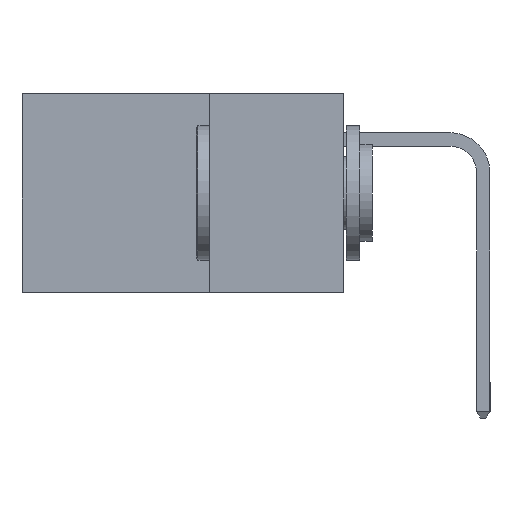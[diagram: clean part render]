
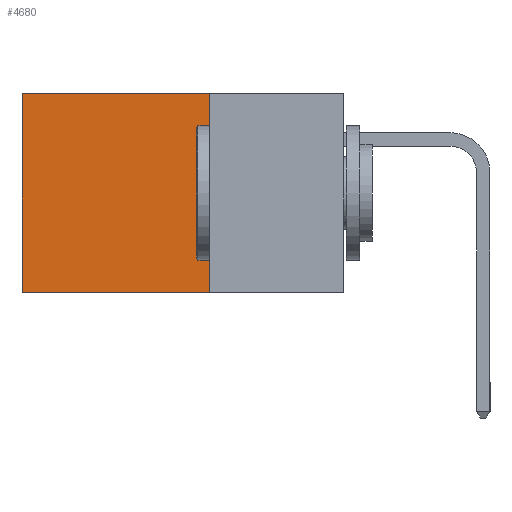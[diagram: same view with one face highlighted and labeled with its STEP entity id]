
A CAD part, left-side view. The second image highlights one B-rep face of the part: STEP entity #4680.
In plain terms, the highlighted planar face has unit normal (-1, 0, 0).
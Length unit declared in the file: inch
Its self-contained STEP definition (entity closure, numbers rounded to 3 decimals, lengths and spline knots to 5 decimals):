
#253 = CARTESIAN_POINT ( 'NONE',  ( 0.298, 0.6, 0. ) ) ;
#821 = VERTEX_POINT ( 'NONE', #8189 ) ;
#877 = ORIENTED_EDGE ( 'NONE', *, *, #25075, .F. ) ;
#981 = VERTEX_POINT ( 'NONE', #253 ) ;
#1596 = EDGE_CURVE ( 'NONE', #12907, #18561, #21260, .T. ) ;
#1654 = ORIENTED_EDGE ( 'NONE', *, *, #10712, .T. ) ;
#2031 = DIRECTION ( 'NONE',  ( 0., 1., 0. ) ) ;
#2987 = PLANE ( 'NONE',  #20745 ) ;
#3049 = CARTESIAN_POINT ( 'NONE',  ( 0.298, 0.6, 0. ) ) ;
#3614 = EDGE_CURVE ( 'NONE', #821, #981, #21253, .T. ) ;
#4680 = ADVANCED_FACE ( 'NONE', ( #14351 ), #2987, .F. ) ;
#4738 = CARTESIAN_POINT ( 'NONE',  ( 0.298, 0.25, -0.37 ) ) ;
#8189 = CARTESIAN_POINT ( 'NONE',  ( 0.298, 0.25, 0. ) ) ;
#8745 = LINE ( 'NONE', #3049, #18729 ) ;
#9806 = VECTOR ( 'NONE', #24701, 39.37008 ) ;
#10047 = VECTOR ( 'NONE', #12560, 39.37008 ) ;
#10699 = VECTOR ( 'NONE', #2031, 39.37008 ) ;
#10712 = EDGE_CURVE ( 'NONE', #981, #18561, #8745, .T. ) ;
#11611 = CARTESIAN_POINT ( 'NONE',  ( 0.298, 0.25, 0. ) ) ;
#12266 = ORIENTED_EDGE ( 'NONE', *, *, #1596, .F. ) ;
#12560 = DIRECTION ( 'NONE',  ( 0., 1., 0. ) ) ;
#12907 = VERTEX_POINT ( 'NONE', #23868 ) ;
#13280 = EDGE_LOOP ( 'NONE', ( #1654, #12266, #877, #16508 ) ) ;
#14351 = FACE_OUTER_BOUND ( 'NONE', #13280, .T. ) ;
#16508 = ORIENTED_EDGE ( 'NONE', *, *, #3614, .T. ) ;
#16931 = DIRECTION ( 'NONE',  ( 0., 0., -1. ) ) ;
#16961 = CARTESIAN_POINT ( 'NONE',  ( 0.298, 0.25, 0. ) ) ;
#17024 = DIRECTION ( 'NONE',  ( 1., 0., 0. ) ) ;
#18561 = VERTEX_POINT ( 'NONE', #19826 ) ;
#18729 = VECTOR ( 'NONE', #16931, 39.37008 ) ;
#19826 = CARTESIAN_POINT ( 'NONE',  ( 0.298, 0.6, -0.37 ) ) ;
#20745 = AXIS2_PLACEMENT_3D ( 'NONE', #11611, #17024, #23879 ) ;
#21253 = LINE ( 'NONE', #16961, #10047 ) ;
#21260 = LINE ( 'NONE', #4738, #10699 ) ;
#22692 = CARTESIAN_POINT ( 'NONE',  ( 0.298, 0.25, 0. ) ) ;
#23868 = CARTESIAN_POINT ( 'NONE',  ( 0.298, 0.25, -0.37 ) ) ;
#23879 = DIRECTION ( 'NONE',  ( 0., 0., -1. ) ) ;
#24701 = DIRECTION ( 'NONE',  ( 0., 0., -1. ) ) ;
#25075 = EDGE_CURVE ( 'NONE', #821, #12907, #25726, .T. ) ;
#25726 = LINE ( 'NONE', #22692, #9806 ) ;
